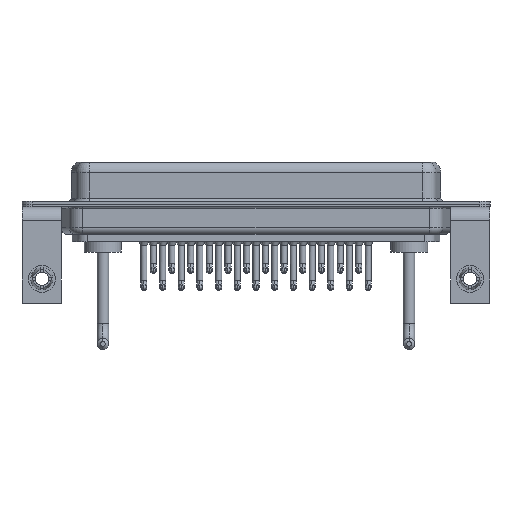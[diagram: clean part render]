
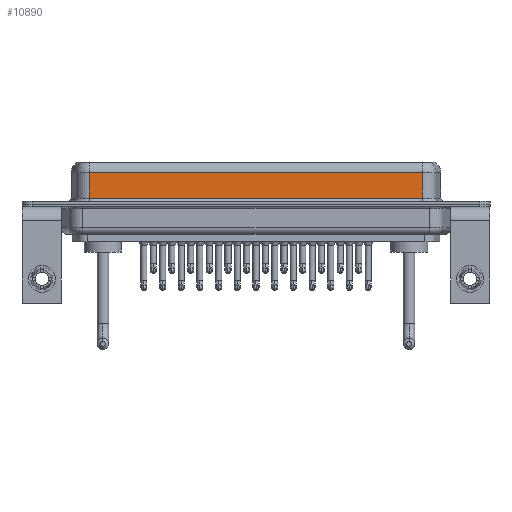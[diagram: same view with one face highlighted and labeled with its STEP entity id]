
A CAD part, front view. The second image highlights one B-rep face of the part: STEP entity #10890.
In plain terms, the highlighted planar face has unit normal (0, -1, 0).
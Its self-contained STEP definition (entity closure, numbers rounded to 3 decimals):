
#8 = DIRECTION ( 'NONE',  ( 0., 0., -1. ) ) ;
#62 = ORIENTED_EDGE ( 'NONE', *, *, #26685, .T. ) ;
#73 = EDGE_CURVE ( 'NONE', #10749, #19343, #24289, .T. ) ;
#1148 = DIRECTION ( 'NONE',  ( 1., 0., 0. ) ) ;
#1519 = CARTESIAN_POINT ( 'NONE',  ( 56.462, -3.95, 6.4 ) ) ;
#4006 = ORIENTED_EDGE ( 'NONE', *, *, #73, .T. ) ;
#4593 = AXIS2_PLACEMENT_3D ( 'NONE', #17105, #8838, #12984 ) ;
#5108 = ORIENTED_EDGE ( 'NONE', *, *, #15200, .T. ) ;
#6247 = FACE_OUTER_BOUND ( 'NONE', #12580, .T. ) ;
#8412 = DIRECTION ( 'NONE',  ( 0., 0., -1. ) ) ;
#8580 = PLANE ( 'NONE',  #4593 ) ;
#8838 = DIRECTION ( 'NONE',  ( 0., 1., 0. ) ) ;
#10716 = ORIENTED_EDGE ( 'NONE', *, *, #22726, .F. ) ;
#10749 = VERTEX_POINT ( 'NONE', #20427 ) ;
#10890 = ADVANCED_FACE ( 'NONE', ( #6247 ), #8580, .F. ) ;
#11373 = VERTEX_POINT ( 'NONE', #14616 ) ;
#12010 = CARTESIAN_POINT ( 'NONE',  ( 56.462, -3.95, 4.65 ) ) ;
#12249 = LINE ( 'NONE', #1519, #17371 ) ;
#12580 = EDGE_LOOP ( 'NONE', ( #10716, #62, #5108, #4006 ) ) ;
#12753 = VERTEX_POINT ( 'NONE', #12010 ) ;
#12984 = DIRECTION ( 'NONE',  ( 0., 0., 1. ) ) ;
#13723 = CARTESIAN_POINT ( 'NONE',  ( 56.462, -3.95, 0.9 ) ) ;
#14616 = CARTESIAN_POINT ( 'NONE',  ( 7.038, -3.95, 4.65 ) ) ;
#14754 = CARTESIAN_POINT ( 'NONE',  ( 7.038, -3.95, 6.4 ) ) ;
#15200 = EDGE_CURVE ( 'NONE', #11373, #10749, #24936, .T. ) ;
#16446 = DIRECTION ( 'NONE',  ( -1., 0., 0. ) ) ;
#17105 = CARTESIAN_POINT ( 'NONE',  ( 56.462, -3.95, 6.4 ) ) ;
#17371 = VECTOR ( 'NONE', #8, 1000. ) ;
#18534 = VECTOR ( 'NONE', #16446, 1000. ) ;
#19343 = VERTEX_POINT ( 'NONE', #13723 ) ;
#19857 = CARTESIAN_POINT ( 'NONE',  ( 56.462, -3.95, 0.9 ) ) ;
#20299 = CARTESIAN_POINT ( 'NONE',  ( 56.462, -3.95, 4.65 ) ) ;
#20427 = CARTESIAN_POINT ( 'NONE',  ( 7.038, -3.95, 0.9 ) ) ;
#21438 = VECTOR ( 'NONE', #8412, 1000. ) ;
#22726 = EDGE_CURVE ( 'NONE', #12753, #19343, #12249, .T. ) ;
#22924 = VECTOR ( 'NONE', #1148, 1000. ) ;
#24289 = LINE ( 'NONE', #19857, #22924 ) ;
#24845 = LINE ( 'NONE', #20299, #18534 ) ;
#24936 = LINE ( 'NONE', #14754, #21438 ) ;
#26685 = EDGE_CURVE ( 'NONE', #12753, #11373, #24845, .T. ) ;
